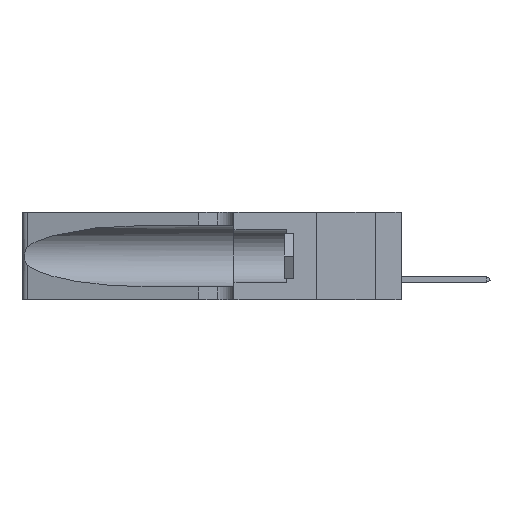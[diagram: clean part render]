
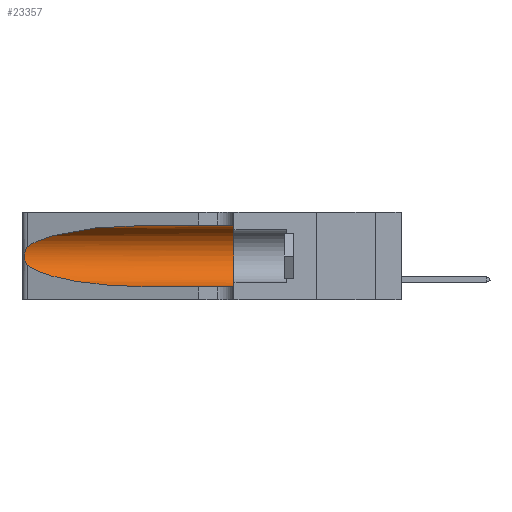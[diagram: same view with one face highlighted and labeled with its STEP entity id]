
A CAD part, left-side view. The second image highlights one B-rep face of the part: STEP entity #23357.
In plain terms, the highlighted cylindrical face has radius 3.308 mm (diameter 6.617 mm), a partial arc.
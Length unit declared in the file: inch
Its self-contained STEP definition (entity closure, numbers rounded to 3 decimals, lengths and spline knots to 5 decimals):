
#2465 = EDGE_LOOP ( 'NONE', ( #29805, #13739, #21606, #30991, #15128, #15617 ) ) ;
#2473 = CARTESIAN_POINT ( 'NONE',  ( 0.2373, 1.15595, 0.08982 ) ) ;
#2839 = CARTESIAN_POINT ( 'NONE',  ( 0.25487, 1.22718, 0.22369 ) ) ;
#3471 = EDGE_CURVE ( 'NONE', #21539, #26663, #26904, .T. ) ;
#3960 = AXIS2_PLACEMENT_3D ( 'NONE', #15011, #17454, #22319 ) ;
#5086 = CYLINDRICAL_SURFACE ( 'NONE', #28232, 0.13025 ) ;
#5225 = CARTESIAN_POINT ( 'NONE',  ( 0.1305, 1.61858, 0.05475 ) ) ;
#5558 = CARTESIAN_POINT ( 'NONE',  ( 0.26075, 1.23896, 0.178 ) ) ;
#5972 = CARTESIAN_POINT ( 'NONE',  ( 0.1305, 1.61858, 0.185 ) ) ;
#6469 = VECTOR ( 'NONE', #13375, 39.37008 ) ;
#8112 = DIRECTION ( 'NONE',  ( 0., -1., 0. ) ) ;
#8139 = CARTESIAN_POINT ( 'NONE',  ( 0.25854, 1.2359, 0.20912 ) ) ;
#8244 = CARTESIAN_POINT ( 'NONE',  ( 0.25639, 1.23186, 0.15144 ) ) ;
#9147 = CARTESIAN_POINT ( 'NONE',  ( 0.25487, 1.22718, 0.22369 ) ) ;
#9593 = VERTEX_POINT ( 'NONE', #14316 ) ;
#9895 = LINE ( 'NONE', #5225, #10271 ) ;
#10271 = VECTOR ( 'NONE', #8112, 39.37008 ) ;
#10434 = CARTESIAN_POINT ( 'NONE',  ( 0.1305, 0.72297, 0.31525 ) ) ;
#10807 = FACE_OUTER_BOUND ( 'NONE', #2465, .T. ) ;
#10894 = CARTESIAN_POINT ( 'NONE',  ( 0.26075, 1.23896, 0.19203 ) ) ;
#12947 = EDGE_CURVE ( 'NONE', #26663, #27609, #16623, .T. ) ;
#13019 = CARTESIAN_POINT ( 'NONE',  ( 0.25856, 1.23593, 0.16098 ) ) ;
#13223 = CARTESIAN_POINT ( 'NONE',  ( 0.25487, 1.22718, 0.22369 ) ) ;
#13375 = DIRECTION ( 'NONE',  ( 0., -1., 0. ) ) ;
#13739 = ORIENTED_EDGE ( 'NONE', *, *, #12947, .T. ) ;
#14316 = CARTESIAN_POINT ( 'NONE',  ( 0.1305, 0.35, 0.05475 ) ) ;
#14723 = EDGE_CURVE ( 'NONE', #22339, #9593, #9895, .T. ) ;
#15011 = CARTESIAN_POINT ( 'NONE',  ( 0.1305, 0.35, 0.185 ) ) ;
#15128 = ORIENTED_EDGE ( 'NONE', *, *, #18733, .F. ) ;
#15466 = CARTESIAN_POINT ( 'NONE',  ( 0.25555, 1.22993, 0.14849 ) ) ;
#15602 = LINE ( 'NONE', #20588, #6469 ) ;
#15617 = ORIENTED_EDGE ( 'NONE', *, *, #25928, .F. ) ;
#15671 = CARTESIAN_POINT ( 'NONE',  ( 0.26017, 1.23833, 0.17102 ) ) ;
#15765 = DIRECTION ( 'NONE',  ( 0., -1., 0. ) ) ;
#16623 = B_SPLINE_CURVE_WITH_KNOTS ( 'NONE', 3,
 ( #13223, #23001, #20231, #25427, #8139, #20122, #10894, #5558, #15671, #13019, #29967, #8244, #15466, #17913 ),
 .UNSPECIFIED., .F., .F.,
 ( 4, 2, 2, 2, 2, 2, 4 ),
 ( 0., 0.00027, 0.00053, 0.00107, 0.0016, 0.00187, 0.00214 ),
 .UNSPECIFIED. ) ;
#17137 = VERTEX_POINT ( 'NONE', #20459 ) ;
#17454 = DIRECTION ( 'NONE',  ( 0., 1., 0. ) ) ;
#17472 = CARTESIAN_POINT ( 'NONE',  ( 0.2373, 1.15595, 0.28018 ) ) ;
#17913 = CARTESIAN_POINT ( 'NONE',  ( 0.25487, 1.22718, 0.14631 ) ) ;
#18733 = EDGE_CURVE ( 'NONE', #17137, #9593, #19458, .T. ) ;
#19408 = CARTESIAN_POINT ( 'NONE',  ( 0.1305, 0.72297, 0.05475 ) ) ;
#19458 = CIRCLE ( 'NONE', #3960, 0.13025 ) ;
#19795 = CARTESIAN_POINT ( 'NONE',  ( 0.18966, 0.96281, 0.31525 ) ) ;
#20122 = CARTESIAN_POINT ( 'NONE',  ( 0.26018, 1.23835, 0.19895 ) ) ;
#20231 = CARTESIAN_POINT ( 'NONE',  ( 0.25639, 1.23184, 0.21858 ) ) ;
#20459 = CARTESIAN_POINT ( 'NONE',  ( 0.1305, 0.35, 0.31525 ) ) ;
#20588 = CARTESIAN_POINT ( 'NONE',  ( 0.1305, 1.61858, 0.31525 ) ) ;
#20645 = DIRECTION ( 'NONE',  ( 0., 0., -1. ) ) ;
#21539 = VERTEX_POINT ( 'NONE', #29107 ) ;
#21606 = ORIENTED_EDGE ( 'NONE', *, *, #29890, .T. ) ;
#21936 = CARTESIAN_POINT ( 'NONE',  ( 0.25487, 1.22718, 0.14631 ) ) ;
#22079 = CARTESIAN_POINT ( 'NONE',  ( 0.25487, 1.22718, 0.14631 ) ) ;
#22319 = DIRECTION ( 'NONE',  ( 0., 0., 1. ) ) ;
#22339 = VERTEX_POINT ( 'NONE', #19408 ) ;
#23001 = CARTESIAN_POINT ( 'NONE',  ( 0.25555, 1.22994, 0.2215 ) ) ;
#23357 = ADVANCED_FACE ( 'NONE', ( #10807 ), #5086, .F. ) ;
#25427 = CARTESIAN_POINT ( 'NONE',  ( 0.25787, 1.23484, 0.2124 ) ) ;
#25928 = EDGE_CURVE ( 'NONE', #21539, #17137, #15602, .T. ) ;
#26663 = VERTEX_POINT ( 'NONE', #9147 ) ;
#26904 =( BOUNDED_CURVE ( )  B_SPLINE_CURVE ( 3, ( #10434, #19795, #17472, #2839 ),
 .UNSPECIFIED., .F., .F. ) 
 B_SPLINE_CURVE_WITH_KNOTS ( ( 4, 4 ),
 ( 1.5708, 2.84003 ),
 .UNSPECIFIED. ) 
 CURVE ( )  GEOMETRIC_REPRESENTATION_ITEM ( )  RATIONAL_B_SPLINE_CURVE ( ( 1., 0.87, 0.87, 1. ) ) 
 REPRESENTATION_ITEM ( '' )  );
#27482 =( BOUNDED_CURVE ( )  B_SPLINE_CURVE ( 3, ( #22079, #2473, #29261, #28961 ),
 .UNSPECIFIED., .F., .F. ) 
 B_SPLINE_CURVE_WITH_KNOTS ( ( 4, 4 ),
 ( 3.44316, 4.71239 ),
 .UNSPECIFIED. ) 
 CURVE ( )  GEOMETRIC_REPRESENTATION_ITEM ( )  RATIONAL_B_SPLINE_CURVE ( ( 1., 0.87, 0.87, 1. ) ) 
 REPRESENTATION_ITEM ( '' )  );
#27609 = VERTEX_POINT ( 'NONE', #21936 ) ;
#28232 = AXIS2_PLACEMENT_3D ( 'NONE', #5972, #15765, #20645 ) ;
#28961 = CARTESIAN_POINT ( 'NONE',  ( 0.1305, 0.72297, 0.05475 ) ) ;
#29107 = CARTESIAN_POINT ( 'NONE',  ( 0.1305, 0.72297, 0.31525 ) ) ;
#29261 = CARTESIAN_POINT ( 'NONE',  ( 0.18966, 0.96281, 0.05475 ) ) ;
#29805 = ORIENTED_EDGE ( 'NONE', *, *, #3471, .T. ) ;
#29890 = EDGE_CURVE ( 'NONE', #27609, #22339, #27482, .T. ) ;
#29967 = CARTESIAN_POINT ( 'NONE',  ( 0.25789, 1.23486, 0.15765 ) ) ;
#30991 = ORIENTED_EDGE ( 'NONE', *, *, #14723, .T. ) ;
